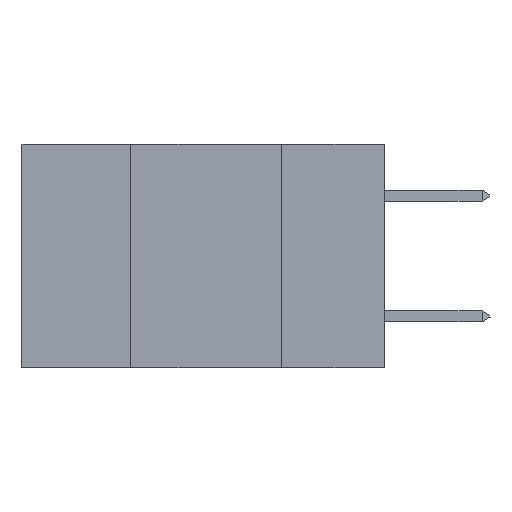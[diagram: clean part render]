
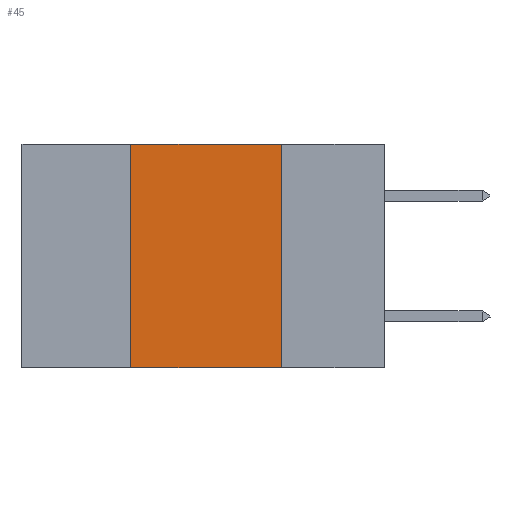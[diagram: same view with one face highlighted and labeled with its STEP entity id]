
A CAD part, left-side view. The second image highlights one B-rep face of the part: STEP entity #45.
In plain terms, the highlighted planar face has unit normal (-1, 0, 0).
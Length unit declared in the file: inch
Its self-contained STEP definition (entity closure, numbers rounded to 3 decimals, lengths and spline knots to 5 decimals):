
#45 = ADVANCED_FACE ( 'NONE', ( #24585 ), #22751, .F. ) ;
#888 = LINE ( 'NONE', #9761, #24578 ) ;
#1194 = DIRECTION ( 'NONE',  ( 0., -1., 0. ) ) ;
#1670 = CARTESIAN_POINT ( 'NONE',  ( 0., 0.6, 0. ) ) ;
#1762 = VERTEX_POINT ( 'NONE', #13925 ) ;
#2515 = EDGE_CURVE ( 'NONE', #24518, #1762, #888, .T. ) ;
#3489 = LINE ( 'NONE', #4970, #12537 ) ;
#3492 = EDGE_CURVE ( 'NONE', #17422, #13461, #10169, .T. ) ;
#3554 = DIRECTION ( 'NONE',  ( 0., 0., -1. ) ) ;
#3630 = DIRECTION ( 'NONE',  ( 1., 0., 0. ) ) ;
#4714 = LINE ( 'NONE', #20639, #6818 ) ;
#4970 = CARTESIAN_POINT ( 'NONE',  ( 0., 0.6, 0. ) ) ;
#6367 = CARTESIAN_POINT ( 'NONE',  ( 0., 0.42, 0. ) ) ;
#6818 = VECTOR ( 'NONE', #15246, 39.37008 ) ;
#7420 = CARTESIAN_POINT ( 'NONE',  ( 0., 0.42, 0. ) ) ;
#8325 = DIRECTION ( 'NONE',  ( 0., 0., 1. ) ) ;
#9761 = CARTESIAN_POINT ( 'NONE',  ( 0., 0.17, 0. ) ) ;
#10169 = LINE ( 'NONE', #6367, #23652 ) ;
#11030 = EDGE_CURVE ( 'NONE', #17422, #1762, #4714, .T. ) ;
#11328 = CARTESIAN_POINT ( 'NONE',  ( 0., 0.17, 0. ) ) ;
#11545 = EDGE_CURVE ( 'NONE', #13461, #24518, #3489, .T. ) ;
#11947 = ORIENTED_EDGE ( 'NONE', *, *, #2515, .F. ) ;
#12174 = EDGE_LOOP ( 'NONE', ( #11947, #24318, #12907, #12521 ) ) ;
#12521 = ORIENTED_EDGE ( 'NONE', *, *, #11030, .T. ) ;
#12537 = VECTOR ( 'NONE', #1194, 39.37008 ) ;
#12907 = ORIENTED_EDGE ( 'NONE', *, *, #3492, .F. ) ;
#13461 = VERTEX_POINT ( 'NONE', #7420 ) ;
#13925 = CARTESIAN_POINT ( 'NONE',  ( 0., 0.17, -0.37 ) ) ;
#15246 = DIRECTION ( 'NONE',  ( 0., -1., 0. ) ) ;
#15302 = DIRECTION ( 'NONE',  ( 0., 0., -1. ) ) ;
#15429 = AXIS2_PLACEMENT_3D ( 'NONE', #1670, #3630, #3554 ) ;
#17422 = VERTEX_POINT ( 'NONE', #20058 ) ;
#20058 = CARTESIAN_POINT ( 'NONE',  ( 0., 0.42, -0.37 ) ) ;
#20639 = CARTESIAN_POINT ( 'NONE',  ( 0., 0.6, -0.37 ) ) ;
#22751 = PLANE ( 'NONE',  #15429 ) ;
#23652 = VECTOR ( 'NONE', #8325, 39.37008 ) ;
#24318 = ORIENTED_EDGE ( 'NONE', *, *, #11545, .F. ) ;
#24518 = VERTEX_POINT ( 'NONE', #11328 ) ;
#24578 = VECTOR ( 'NONE', #15302, 39.37008 ) ;
#24585 = FACE_OUTER_BOUND ( 'NONE', #12174, .T. ) ;
